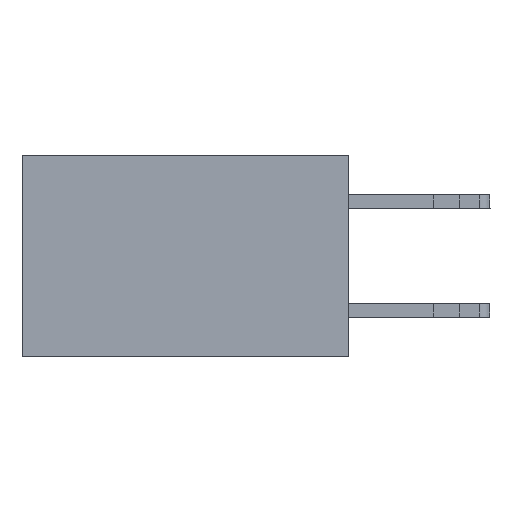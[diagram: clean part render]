
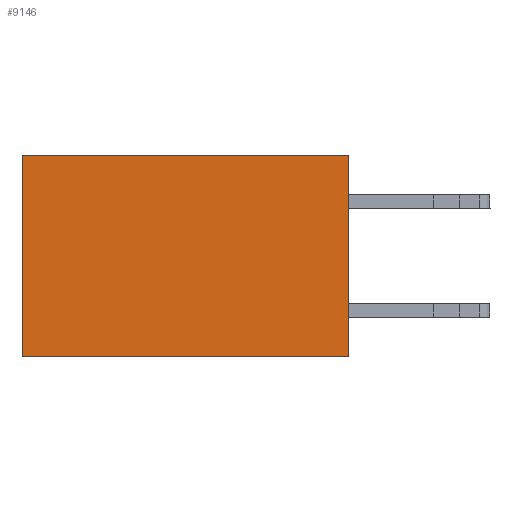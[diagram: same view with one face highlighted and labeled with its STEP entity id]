
A CAD part, left-side view. The second image highlights one B-rep face of the part: STEP entity #9146.
In plain terms, the highlighted planar face has unit normal (-1, 0, 0).
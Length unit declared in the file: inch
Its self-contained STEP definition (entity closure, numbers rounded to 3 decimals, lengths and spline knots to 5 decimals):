
#316 = VERTEX_POINT ( 'NONE', #3377 ) ;
#854 = CARTESIAN_POINT ( 'NONE',  ( 0.2615, 0., 0. ) ) ;
#911 = ORIENTED_EDGE ( 'NONE', *, *, #10361, .F. ) ;
#1852 = DIRECTION ( 'NONE',  ( 0., 0., -1. ) ) ;
#2665 = PLANE ( 'NONE',  #4286 ) ;
#3177 = DIRECTION ( 'NONE',  ( 0., 0., -1. ) ) ;
#3377 = CARTESIAN_POINT ( 'NONE',  ( 0.2615, 0.6, 0. ) ) ;
#3385 = EDGE_CURVE ( 'NONE', #316, #12002, #11725, .T. ) ;
#3622 = CARTESIAN_POINT ( 'NONE',  ( 0.2615, 0.6, -0.37 ) ) ;
#3881 = VECTOR ( 'NONE', #6928, 39.37008 ) ;
#4286 = AXIS2_PLACEMENT_3D ( 'NONE', #5540, #7769, #1852 ) ;
#4563 = CARTESIAN_POINT ( 'NONE',  ( 0.2615, 0., -0.37 ) ) ;
#5141 = CARTESIAN_POINT ( 'NONE',  ( 0.2615, 0.6, -0.37 ) ) ;
#5383 = VERTEX_POINT ( 'NONE', #11807 ) ;
#5540 = CARTESIAN_POINT ( 'NONE',  ( 0.2615, 0., -0.37 ) ) ;
#6106 = CARTESIAN_POINT ( 'NONE',  ( 0.2615, 0., -0.37 ) ) ;
#6677 = ORIENTED_EDGE ( 'NONE', *, *, #3385, .T. ) ;
#6725 = VERTEX_POINT ( 'NONE', #4563 ) ;
#6928 = DIRECTION ( 'NONE',  ( 0., 1., 0. ) ) ;
#6997 = DIRECTION ( 'NONE',  ( 0., 0., -1. ) ) ;
#7523 = LINE ( 'NONE', #854, #11637 ) ;
#7714 = DIRECTION ( 'NONE',  ( 0., 1., 0. ) ) ;
#7769 = DIRECTION ( 'NONE',  ( 1., 0., 0. ) ) ;
#7827 = VECTOR ( 'NONE', #6997, 39.37008 ) ;
#7860 = VECTOR ( 'NONE', #3177, 39.37008 ) ;
#7862 = CARTESIAN_POINT ( 'NONE',  ( 0.2615, 0., -0.37 ) ) ;
#7903 = ORIENTED_EDGE ( 'NONE', *, *, #10015, .T. ) ;
#8908 = EDGE_CURVE ( 'NONE', #6725, #12002, #8912, .T. ) ;
#8912 = LINE ( 'NONE', #6106, #3881 ) ;
#9018 = EDGE_LOOP ( 'NONE', ( #6677, #11446, #911, #7903 ) ) ;
#9146 = ADVANCED_FACE ( 'NONE', ( #11202 ), #2665, .F. ) ;
#9675 = LINE ( 'NONE', #7862, #7860 ) ;
#10015 = EDGE_CURVE ( 'NONE', #5383, #316, #7523, .T. ) ;
#10361 = EDGE_CURVE ( 'NONE', #5383, #6725, #9675, .T. ) ;
#11202 = FACE_OUTER_BOUND ( 'NONE', #9018, .T. ) ;
#11446 = ORIENTED_EDGE ( 'NONE', *, *, #8908, .F. ) ;
#11637 = VECTOR ( 'NONE', #7714, 39.37008 ) ;
#11725 = LINE ( 'NONE', #5141, #7827 ) ;
#11807 = CARTESIAN_POINT ( 'NONE',  ( 0.2615, 0., 0. ) ) ;
#12002 = VERTEX_POINT ( 'NONE', #3622 ) ;
